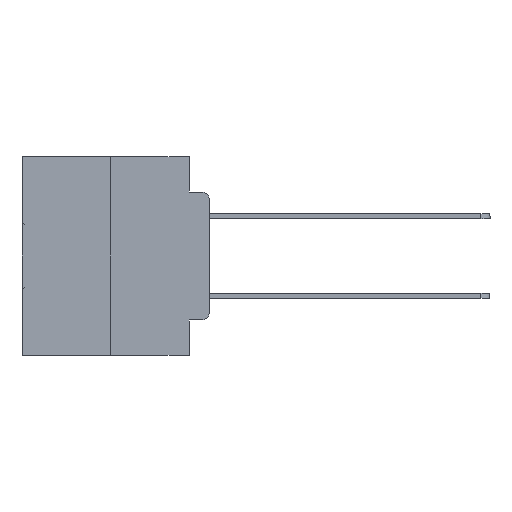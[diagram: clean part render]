
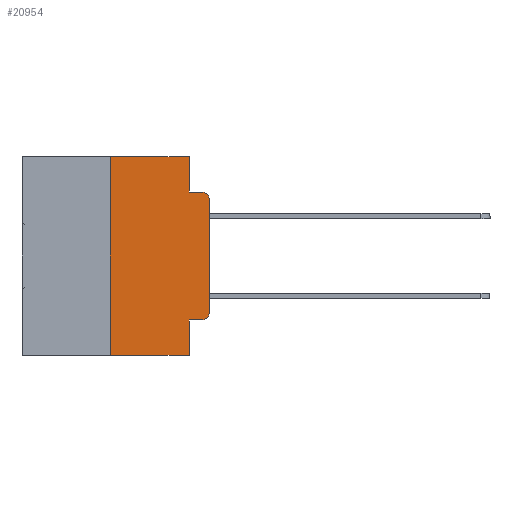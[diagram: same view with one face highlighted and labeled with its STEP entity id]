
A CAD part, left-side view. The second image highlights one B-rep face of the part: STEP entity #20954.
In plain terms, the highlighted planar face has unit normal (-1, 0, 0).
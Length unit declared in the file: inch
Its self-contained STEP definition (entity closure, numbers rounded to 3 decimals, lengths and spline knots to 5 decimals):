
#489 = CARTESIAN_POINT ( 'NONE',  ( 0., 0.473, 0. ) ) ;
#804 = CARTESIAN_POINT ( 'NONE',  ( 0., 0.051, -0.0885 ) ) ;
#1470 = LINE ( 'NONE', #22986, #27674 ) ;
#2207 = DIRECTION ( 'NONE',  ( -1., 0., 0. ) ) ;
#2377 = VERTEX_POINT ( 'NONE', #13223 ) ;
#2467 = AXIS2_PLACEMENT_3D ( 'NONE', #17533, #2207, #20074 ) ;
#3061 = DIRECTION ( 'NONE',  ( 0., -1., 0. ) ) ;
#3362 = CARTESIAN_POINT ( 'NONE',  ( 0., 0.02, -0.3915 ) ) ;
#4171 = VERTEX_POINT ( 'NONE', #28084 ) ;
#5078 = DIRECTION ( 'NONE',  ( 0., 0., 1. ) ) ;
#5642 = CARTESIAN_POINT ( 'NONE',  ( 0., 0.473, 0. ) ) ;
#5874 = AXIS2_PLACEMENT_3D ( 'NONE', #3362, #21218, #5981 ) ;
#5981 = DIRECTION ( 'NONE',  ( 0., 0., -1. ) ) ;
#6710 = CARTESIAN_POINT ( 'NONE',  ( 0., 0.051, -0.0885 ) ) ;
#6765 = ORIENTED_EDGE ( 'NONE', *, *, #17000, .T. ) ;
#6969 = EDGE_CURVE ( 'NONE', #4171, #2377, #11142, .T. ) ;
#7240 = VECTOR ( 'NONE', #32564, 39.37008 ) ;
#7658 = CARTESIAN_POINT ( 'NONE',  ( 0., 0.25, 0. ) ) ;
#7791 = ORIENTED_EDGE ( 'NONE', *, *, #17203, .F. ) ;
#8023 = ORIENTED_EDGE ( 'NONE', *, *, #24088, .F. ) ;
#8216 = DIRECTION ( 'NONE',  ( 0., 0., -1. ) ) ;
#8494 = ORIENTED_EDGE ( 'NONE', *, *, #18899, .F. ) ;
#8512 = AXIS2_PLACEMENT_3D ( 'NONE', #5642, #23425, #8216 ) ;
#8865 = EDGE_LOOP ( 'NONE', ( #11285, #11165, #9978, #8494, #8023, #7791, #6765, #29486, #17491, #23387 ) ) ;
#9465 = CARTESIAN_POINT ( 'NONE',  ( 0., 0.473, -0.5 ) ) ;
#9603 = VECTOR ( 'NONE', #12038, 39.37008 ) ;
#9782 = VERTEX_POINT ( 'NONE', #22138 ) ;
#9978 = ORIENTED_EDGE ( 'NONE', *, *, #25630, .F. ) ;
#10429 = LINE ( 'NONE', #9465, #9603 ) ;
#10975 = CIRCLE ( 'NONE', #2467, 0.02 ) ;
#11142 = CIRCLE ( 'NONE', #5874, 0.02 ) ;
#11153 = CARTESIAN_POINT ( 'NONE',  ( 0., 0.25, -0.5 ) ) ;
#11165 = ORIENTED_EDGE ( 'NONE', *, *, #28950, .T. ) ;
#11285 = ORIENTED_EDGE ( 'NONE', *, *, #30597, .T. ) ;
#11755 = VECTOR ( 'NONE', #14019, 39.37008 ) ;
#12038 = DIRECTION ( 'NONE',  ( 0., -1., 0. ) ) ;
#12903 = VERTEX_POINT ( 'NONE', #21487 ) ;
#13223 = CARTESIAN_POINT ( 'NONE',  ( 0., 0., -0.3915 ) ) ;
#13779 = EDGE_CURVE ( 'NONE', #12903, #4171, #15369, .T. ) ;
#13918 = CARTESIAN_POINT ( 'NONE',  ( 0., 0.051, 0. ) ) ;
#14019 = DIRECTION ( 'NONE',  ( 0., 0., -1. ) ) ;
#15369 = LINE ( 'NONE', #19882, #20519 ) ;
#15492 = EDGE_CURVE ( 'NONE', #12903, #9782, #31730, .T. ) ;
#15570 = VERTEX_POINT ( 'NONE', #26238 ) ;
#15780 = PLANE ( 'NONE',  #8512 ) ;
#17000 = EDGE_CURVE ( 'NONE', #32027, #9782, #10429, .T. ) ;
#17203 = EDGE_CURVE ( 'NONE', #32027, #30194, #17552, .T. ) ;
#17491 = ORIENTED_EDGE ( 'NONE', *, *, #13779, .T. ) ;
#17533 = CARTESIAN_POINT ( 'NONE',  ( 0., 0.02, -0.1085 ) ) ;
#17552 = LINE ( 'NONE', #7658, #30058 ) ;
#17668 = CARTESIAN_POINT ( 'NONE',  ( 0., 0., 0. ) ) ;
#18899 = EDGE_CURVE ( 'NONE', #29404, #27133, #1470, .T. ) ;
#19275 = CARTESIAN_POINT ( 'NONE',  ( 0., 0.051, 0. ) ) ;
#19598 = LINE ( 'NONE', #804, #32032 ) ;
#19657 = VECTOR ( 'NONE', #3061, 39.37008 ) ;
#19882 = CARTESIAN_POINT ( 'NONE',  ( 0., 0.051, -0.4115 ) ) ;
#20074 = DIRECTION ( 'NONE',  ( 0., 0., -1. ) ) ;
#20519 = VECTOR ( 'NONE', #22412, 39.37008 ) ;
#20755 = LINE ( 'NONE', #17668, #7240 ) ;
#20954 = ADVANCED_FACE ( 'NONE', ( #32299 ), #15780, .F. ) ;
#21218 = DIRECTION ( 'NONE',  ( -1., 0., 0. ) ) ;
#21245 = DIRECTION ( 'NONE',  ( 0., -1., 0. ) ) ;
#21487 = CARTESIAN_POINT ( 'NONE',  ( 0., 0.051, -0.4115 ) ) ;
#22138 = CARTESIAN_POINT ( 'NONE',  ( 0., 0.051, -0.5 ) ) ;
#22412 = DIRECTION ( 'NONE',  ( 0., -1., 0. ) ) ;
#22986 = CARTESIAN_POINT ( 'NONE',  ( 0., 0.051, 0. ) ) ;
#23387 = ORIENTED_EDGE ( 'NONE', *, *, #6969, .T. ) ;
#23425 = DIRECTION ( 'NONE',  ( 1., 0., 0. ) ) ;
#24088 = EDGE_CURVE ( 'NONE', #30194, #29404, #26329, .T. ) ;
#25630 = EDGE_CURVE ( 'NONE', #27133, #27485, #19598, .T. ) ;
#26196 = CARTESIAN_POINT ( 'NONE',  ( 0., 0.02, -0.0885 ) ) ;
#26238 = CARTESIAN_POINT ( 'NONE',  ( 0., 0., -0.1085 ) ) ;
#26329 = LINE ( 'NONE', #489, #19657 ) ;
#27133 = VERTEX_POINT ( 'NONE', #6710 ) ;
#27485 = VERTEX_POINT ( 'NONE', #26196 ) ;
#27674 = VECTOR ( 'NONE', #27975, 39.37008 ) ;
#27975 = DIRECTION ( 'NONE',  ( 0., 0., -1. ) ) ;
#28084 = CARTESIAN_POINT ( 'NONE',  ( 0., 0.02, -0.4115 ) ) ;
#28514 = CARTESIAN_POINT ( 'NONE',  ( 0., 0.25, 0. ) ) ;
#28950 = EDGE_CURVE ( 'NONE', #15570, #27485, #10975, .T. ) ;
#29404 = VERTEX_POINT ( 'NONE', #19275 ) ;
#29486 = ORIENTED_EDGE ( 'NONE', *, *, #15492, .F. ) ;
#30058 = VECTOR ( 'NONE', #5078, 39.37008 ) ;
#30194 = VERTEX_POINT ( 'NONE', #28514 ) ;
#30597 = EDGE_CURVE ( 'NONE', #2377, #15570, #20755, .T. ) ;
#31730 = LINE ( 'NONE', #13918, #11755 ) ;
#32027 = VERTEX_POINT ( 'NONE', #11153 ) ;
#32032 = VECTOR ( 'NONE', #21245, 39.37008 ) ;
#32299 = FACE_OUTER_BOUND ( 'NONE', #8865, .T. ) ;
#32564 = DIRECTION ( 'NONE',  ( 0., 0., 1. ) ) ;
